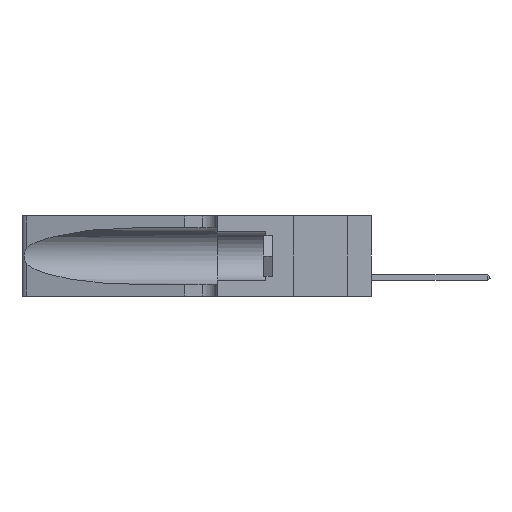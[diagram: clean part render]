
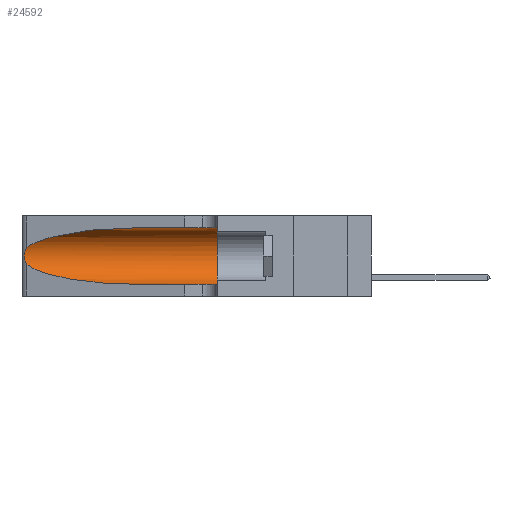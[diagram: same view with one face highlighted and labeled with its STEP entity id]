
A CAD part, left-side view. The second image highlights one B-rep face of the part: STEP entity #24592.
In plain terms, the highlighted cylindrical face has radius 3.308 mm (diameter 6.617 mm), a partial arc.
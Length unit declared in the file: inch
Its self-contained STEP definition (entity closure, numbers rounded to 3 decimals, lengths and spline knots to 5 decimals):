
#1842 = VERTEX_POINT ( 'NONE', #4238 ) ;
#1854 = DIRECTION ( 'NONE',  ( 0., -1., 0. ) ) ;
#2012 = FACE_OUTER_BOUND ( 'NONE', #22285, .T. ) ;
#2731 = AXIS2_PLACEMENT_3D ( 'NONE', #23173, #1854, #20689 ) ;
#3783 = EDGE_CURVE ( 'NONE', #25140, #15620, #18516, .T. ) ;
#3920 = CARTESIAN_POINT ( 'NONE',  ( 0.25787, 1.23484, 0.2124 ) ) ;
#4238 = CARTESIAN_POINT ( 'NONE',  ( 0.1305, 0.72297, 0.05475 ) ) ;
#4999 = CARTESIAN_POINT ( 'NONE',  ( 0.25487, 1.22718, 0.22369 ) ) ;
#5104 = DIRECTION ( 'NONE',  ( 0., 0., 1. ) ) ;
#5193 = VERTEX_POINT ( 'NONE', #5471 ) ;
#5448 = DIRECTION ( 'NONE',  ( 0., 1., 0. ) ) ;
#5471 = CARTESIAN_POINT ( 'NONE',  ( 0.1305, 0.35, 0.05475 ) ) ;
#6181 = ORIENTED_EDGE ( 'NONE', *, *, #32257, .T. ) ;
#7265 = CARTESIAN_POINT ( 'NONE',  ( 0.1305, 1.61858, 0.05475 ) ) ;
#7431 = CARTESIAN_POINT ( 'NONE',  ( 0.25856, 1.23593, 0.16098 ) ) ;
#7516 = DIRECTION ( 'NONE',  ( 0., -1., 0. ) ) ;
#7786 = CARTESIAN_POINT ( 'NONE',  ( 0.26017, 1.23833, 0.17102 ) ) ;
#7892 = ORIENTED_EDGE ( 'NONE', *, *, #17024, .F. ) ;
#9608 = EDGE_CURVE ( 'NONE', #18305, #30579, #28703, .T. ) ;
#10634 = CARTESIAN_POINT ( 'NONE',  ( 0.1305, 0.35, 0.185 ) ) ;
#10830 = CARTESIAN_POINT ( 'NONE',  ( 0.25555, 1.22994, 0.2215 ) ) ;
#11076 = ORIENTED_EDGE ( 'NONE', *, *, #3783, .T. ) ;
#12207 =( BOUNDED_CURVE ( )  B_SPLINE_CURVE ( 3, ( #15427, #26607, #18124, #4999 ),
 .UNSPECIFIED., .F., .F. ) 
 B_SPLINE_CURVE_WITH_KNOTS ( ( 4, 4 ),
 ( 1.5708, 2.84003 ),
 .UNSPECIFIED. ) 
 CURVE ( )  GEOMETRIC_REPRESENTATION_ITEM ( )  RATIONAL_B_SPLINE_CURVE ( ( 1., 0.87, 0.87, 1. ) ) 
 REPRESENTATION_ITEM ( '' )  );
#12430 = ORIENTED_EDGE ( 'NONE', *, *, #9608, .F. ) ;
#12809 = EDGE_CURVE ( 'NONE', #18305, #25140, #12207, .T. ) ;
#12912 = CARTESIAN_POINT ( 'NONE',  ( 0.25789, 1.23486, 0.15765 ) ) ;
#13134 = CARTESIAN_POINT ( 'NONE',  ( 0.25487, 1.22718, 0.14631 ) ) ;
#13566 = CARTESIAN_POINT ( 'NONE',  ( 0.25639, 1.23184, 0.21858 ) ) ;
#13791 = CARTESIAN_POINT ( 'NONE',  ( 0.2373, 1.15595, 0.08982 ) ) ;
#14959 = CARTESIAN_POINT ( 'NONE',  ( 0.25487, 1.22718, 0.22369 ) ) ;
#15427 = CARTESIAN_POINT ( 'NONE',  ( 0.1305, 0.72297, 0.31525 ) ) ;
#15620 = VERTEX_POINT ( 'NONE', #13134 ) ;
#15694 = LINE ( 'NONE', #7265, #18625 ) ;
#15920 =( BOUNDED_CURVE ( )  B_SPLINE_CURVE ( 3, ( #29871, #13791, #16494, #27020 ),
 .UNSPECIFIED., .F., .T. ) 
 B_SPLINE_CURVE_WITH_KNOTS ( ( 4, 4 ),
 ( 3.44316, 4.71239 ),
 .UNSPECIFIED. ) 
 CURVE ( )  GEOMETRIC_REPRESENTATION_ITEM ( )  RATIONAL_B_SPLINE_CURVE ( ( 1., 0.87, 0.87, 1. ) ) 
 REPRESENTATION_ITEM ( '' )  );
#16193 = CARTESIAN_POINT ( 'NONE',  ( 0.1305, 1.61858, 0.31525 ) ) ;
#16494 = CARTESIAN_POINT ( 'NONE',  ( 0.18966, 0.96281, 0.05475 ) ) ;
#16736 = DIRECTION ( 'NONE',  ( 0., -1., 0. ) ) ;
#17024 = EDGE_CURVE ( 'NONE', #30579, #5193, #26155, .T. ) ;
#18124 = CARTESIAN_POINT ( 'NONE',  ( 0.2373, 1.15595, 0.28018 ) ) ;
#18305 = VERTEX_POINT ( 'NONE', #19287 ) ;
#18315 = CARTESIAN_POINT ( 'NONE',  ( 0.25487, 1.22718, 0.22369 ) ) ;
#18516 = B_SPLINE_CURVE_WITH_KNOTS ( 'NONE', 3,
 ( #18315, #10830, #13566, #3920, #33812, #31575, #24062, #23820, #7786, #7431, #12912, #31923, #27496, #32375 ),
 .UNSPECIFIED., .F., .F.,
 ( 4, 2, 2, 2, 2, 2, 4 ),
 ( 0., 0.00027, 0.00053, 0.00107, 0.0016, 0.00187, 0.00214 ),
 .UNSPECIFIED. ) ;
#18625 = VECTOR ( 'NONE', #7516, 39.37008 ) ;
#19287 = CARTESIAN_POINT ( 'NONE',  ( 0.1305, 0.72297, 0.31525 ) ) ;
#19739 = CYLINDRICAL_SURFACE ( 'NONE', #2731, 0.13025 ) ;
#20689 = DIRECTION ( 'NONE',  ( 0., 0., -1. ) ) ;
#21436 = VECTOR ( 'NONE', #16736, 39.37008 ) ;
#22204 = EDGE_CURVE ( 'NONE', #1842, #5193, #15694, .T. ) ;
#22285 = EDGE_LOOP ( 'NONE', ( #28954, #11076, #6181, #27254, #7892, #12430 ) ) ;
#22772 = CARTESIAN_POINT ( 'NONE',  ( 0.1305, 0.35, 0.31525 ) ) ;
#23173 = CARTESIAN_POINT ( 'NONE',  ( 0.1305, 1.61858, 0.185 ) ) ;
#23236 = AXIS2_PLACEMENT_3D ( 'NONE', #10634, #5448, #5104 ) ;
#23820 = CARTESIAN_POINT ( 'NONE',  ( 0.26075, 1.23896, 0.178 ) ) ;
#24062 = CARTESIAN_POINT ( 'NONE',  ( 0.26075, 1.23896, 0.19203 ) ) ;
#24592 = ADVANCED_FACE ( 'NONE', ( #2012 ), #19739, .F. ) ;
#25140 = VERTEX_POINT ( 'NONE', #14959 ) ;
#26155 = CIRCLE ( 'NONE', #23236, 0.13025 ) ;
#26607 = CARTESIAN_POINT ( 'NONE',  ( 0.18966, 0.96281, 0.31525 ) ) ;
#27020 = CARTESIAN_POINT ( 'NONE',  ( 0.1305, 0.72297, 0.05475 ) ) ;
#27254 = ORIENTED_EDGE ( 'NONE', *, *, #22204, .T. ) ;
#27496 = CARTESIAN_POINT ( 'NONE',  ( 0.25555, 1.22993, 0.14849 ) ) ;
#28703 = LINE ( 'NONE', #16193, #21436 ) ;
#28954 = ORIENTED_EDGE ( 'NONE', *, *, #12809, .T. ) ;
#29871 = CARTESIAN_POINT ( 'NONE',  ( 0.25487, 1.22718, 0.14631 ) ) ;
#30579 = VERTEX_POINT ( 'NONE', #22772 ) ;
#31575 = CARTESIAN_POINT ( 'NONE',  ( 0.26018, 1.23835, 0.19895 ) ) ;
#31923 = CARTESIAN_POINT ( 'NONE',  ( 0.25639, 1.23186, 0.15144 ) ) ;
#32257 = EDGE_CURVE ( 'NONE', #15620, #1842, #15920, .T. ) ;
#32375 = CARTESIAN_POINT ( 'NONE',  ( 0.25487, 1.22718, 0.14631 ) ) ;
#33812 = CARTESIAN_POINT ( 'NONE',  ( 0.25854, 1.2359, 0.20912 ) ) ;
